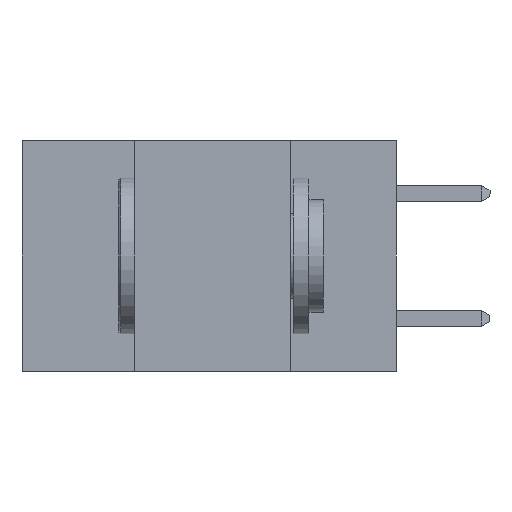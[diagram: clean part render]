
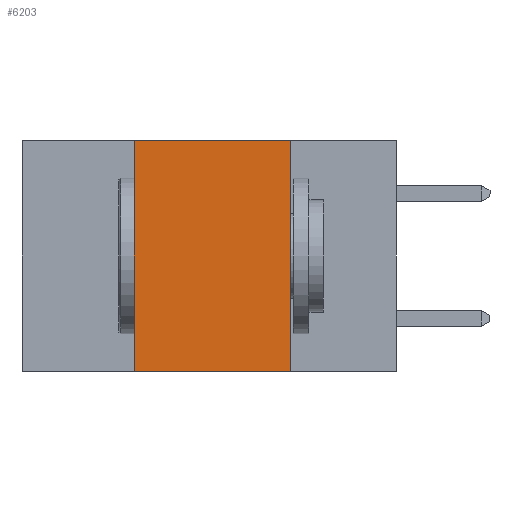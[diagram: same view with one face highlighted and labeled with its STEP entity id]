
A CAD part, left-side view. The second image highlights one B-rep face of the part: STEP entity #6203.
In plain terms, the highlighted planar face has unit normal (-1, 0, 0).
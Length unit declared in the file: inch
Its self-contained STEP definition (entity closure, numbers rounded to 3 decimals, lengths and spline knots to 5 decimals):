
#268 = PLANE ( 'NONE',  #3273 ) ;
#277 = CARTESIAN_POINT ( 'NONE',  ( 0., 0.42, -0.37 ) ) ;
#368 = CARTESIAN_POINT ( 'NONE',  ( 0., 0.17, -0.37 ) ) ;
#413 = VERTEX_POINT ( 'NONE', #917 ) ;
#539 = ORIENTED_EDGE ( 'NONE', *, *, #5979, .F. ) ;
#851 = VECTOR ( 'NONE', #1982, 39.37008 ) ;
#917 = CARTESIAN_POINT ( 'NONE',  ( 0., 0.42, 0. ) ) ;
#970 = CARTESIAN_POINT ( 'NONE',  ( 0., 0.6, 0. ) ) ;
#1218 = CARTESIAN_POINT ( 'NONE',  ( 0., 0.17, 0. ) ) ;
#1302 = CARTESIAN_POINT ( 'NONE',  ( 0., 0.17, -0.37 ) ) ;
#1359 = EDGE_LOOP ( 'NONE', ( #539, #9057, #3734, #7393 ) ) ;
#1421 = EDGE_CURVE ( 'NONE', #5185, #7430, #5312, .T. ) ;
#1982 = DIRECTION ( 'NONE',  ( 0., -1., 0. ) ) ;
#2913 = CARTESIAN_POINT ( 'NONE',  ( 0., 0.6, 0. ) ) ;
#3273 = AXIS2_PLACEMENT_3D ( 'NONE', #970, #6045, #8914 ) ;
#3608 = VECTOR ( 'NONE', #7377, 39.37008 ) ;
#3734 = ORIENTED_EDGE ( 'NONE', *, *, #8648, .F. ) ;
#4164 = VERTEX_POINT ( 'NONE', #1218 ) ;
#4212 = DIRECTION ( 'NONE',  ( 0., 0., -1. ) ) ;
#4653 = EDGE_CURVE ( 'NONE', #413, #4164, #4967, .T. ) ;
#4967 = LINE ( 'NONE', #2913, #851 ) ;
#4970 = LINE ( 'NONE', #1302, #6901 ) ;
#5185 = VERTEX_POINT ( 'NONE', #7525 ) ;
#5295 = FACE_OUTER_BOUND ( 'NONE', #1359, .T. ) ;
#5312 = LINE ( 'NONE', #6671, #6097 ) ;
#5979 = EDGE_CURVE ( 'NONE', #4164, #7430, #4970, .T. ) ;
#6045 = DIRECTION ( 'NONE',  ( 1., 0., 0. ) ) ;
#6097 = VECTOR ( 'NONE', #8181, 39.37008 ) ;
#6203 = ADVANCED_FACE ( 'NONE', ( #5295 ), #268, .F. ) ;
#6671 = CARTESIAN_POINT ( 'NONE',  ( 0., 0.6, -0.37 ) ) ;
#6757 = LINE ( 'NONE', #277, #3608 ) ;
#6901 = VECTOR ( 'NONE', #4212, 39.37008 ) ;
#7377 = DIRECTION ( 'NONE',  ( 0., 0., 1. ) ) ;
#7393 = ORIENTED_EDGE ( 'NONE', *, *, #1421, .T. ) ;
#7430 = VERTEX_POINT ( 'NONE', #368 ) ;
#7525 = CARTESIAN_POINT ( 'NONE',  ( 0., 0.42, -0.37 ) ) ;
#8181 = DIRECTION ( 'NONE',  ( 0., -1., 0. ) ) ;
#8648 = EDGE_CURVE ( 'NONE', #5185, #413, #6757, .T. ) ;
#8914 = DIRECTION ( 'NONE',  ( 0., 0., -1. ) ) ;
#9057 = ORIENTED_EDGE ( 'NONE', *, *, #4653, .F. ) ;
